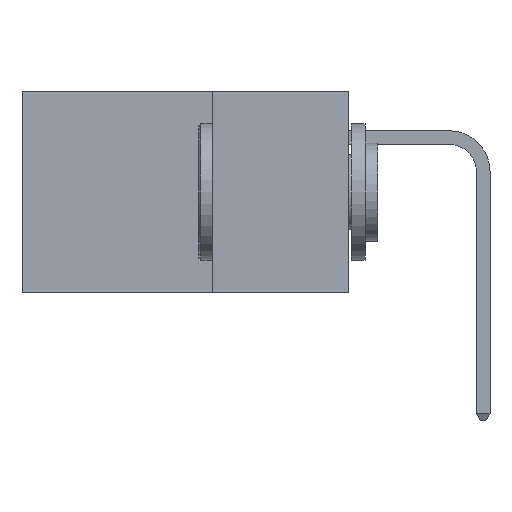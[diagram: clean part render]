
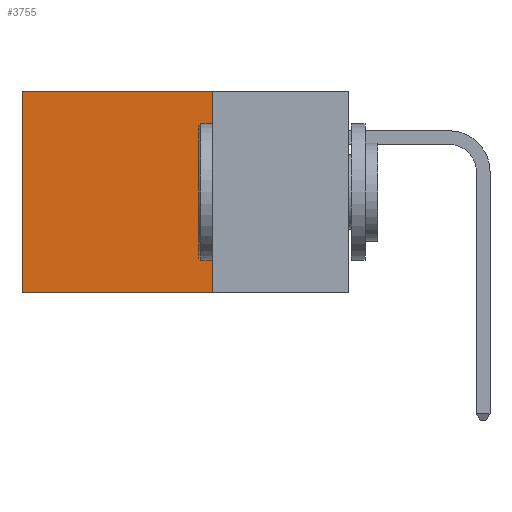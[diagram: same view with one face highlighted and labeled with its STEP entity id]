
A CAD part, left-side view. The second image highlights one B-rep face of the part: STEP entity #3755.
In plain terms, the highlighted planar face has unit normal (-1, 0, 0).
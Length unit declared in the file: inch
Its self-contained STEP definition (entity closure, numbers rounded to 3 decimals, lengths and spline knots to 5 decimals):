
#157 = VECTOR ( 'NONE', #552, 39.37008 ) ;
#552 = DIRECTION ( 'NONE',  ( 0., 0., -1. ) ) ;
#764 = LINE ( 'NONE', #7407, #3009 ) ;
#1059 = LINE ( 'NONE', #9791, #10030 ) ;
#1377 = VERTEX_POINT ( 'NONE', #9768 ) ;
#2729 = DIRECTION ( 'NONE',  ( 1., 0., 0. ) ) ;
#2749 = LINE ( 'NONE', #8305, #157 ) ;
#2848 = ORIENTED_EDGE ( 'NONE', *, *, #8945, .T. ) ;
#2862 = ORIENTED_EDGE ( 'NONE', *, *, #9578, .F. ) ;
#2917 = ORIENTED_EDGE ( 'NONE', *, *, #7736, .F. ) ;
#2971 = ORIENTED_EDGE ( 'NONE', *, *, #7416, .T. ) ;
#3009 = VECTOR ( 'NONE', #3635, 39.37008 ) ;
#3179 = VERTEX_POINT ( 'NONE', #8625 ) ;
#3292 = DIRECTION ( 'NONE',  ( 0., 0., -1. ) ) ;
#3604 = CARTESIAN_POINT ( 'NONE',  ( 0.2875, 0.25, 0. ) ) ;
#3635 = DIRECTION ( 'NONE',  ( 0., 0., -1. ) ) ;
#3755 = ADVANCED_FACE ( 'NONE', ( #9811 ), #4297, .F. ) ;
#4177 = VERTEX_POINT ( 'NONE', #10307 ) ;
#4297 = PLANE ( 'NONE',  #6810 ) ;
#4434 = VECTOR ( 'NONE', #9743, 39.37008 ) ;
#6696 = LINE ( 'NONE', #9763, #4434 ) ;
#6810 = AXIS2_PLACEMENT_3D ( 'NONE', #3604, #2729, #3292 ) ;
#7407 = CARTESIAN_POINT ( 'NONE',  ( 0.2875, 0.6, 0. ) ) ;
#7416 = EDGE_CURVE ( 'NONE', #9437, #3179, #6696, .T. ) ;
#7736 = EDGE_CURVE ( 'NONE', #9437, #4177, #2749, .T. ) ;
#8305 = CARTESIAN_POINT ( 'NONE',  ( 0.2875, 0.25, 0. ) ) ;
#8625 = CARTESIAN_POINT ( 'NONE',  ( 0.2875, 0.6, 0. ) ) ;
#8945 = EDGE_CURVE ( 'NONE', #3179, #1377, #764, .T. ) ;
#9092 = DIRECTION ( 'NONE',  ( 0., 1., 0. ) ) ;
#9230 = EDGE_LOOP ( 'NONE', ( #2848, #2862, #2917, #2971 ) ) ;
#9437 = VERTEX_POINT ( 'NONE', #10327 ) ;
#9578 = EDGE_CURVE ( 'NONE', #4177, #1377, #1059, .T. ) ;
#9743 = DIRECTION ( 'NONE',  ( 0., 1., 0. ) ) ;
#9763 = CARTESIAN_POINT ( 'NONE',  ( 0.2875, 0.25, 0. ) ) ;
#9768 = CARTESIAN_POINT ( 'NONE',  ( 0.2875, 0.6, -0.37 ) ) ;
#9791 = CARTESIAN_POINT ( 'NONE',  ( 0.2875, 0.25, -0.37 ) ) ;
#9811 = FACE_OUTER_BOUND ( 'NONE', #9230, .T. ) ;
#10030 = VECTOR ( 'NONE', #9092, 39.37008 ) ;
#10307 = CARTESIAN_POINT ( 'NONE',  ( 0.2875, 0.25, -0.37 ) ) ;
#10327 = CARTESIAN_POINT ( 'NONE',  ( 0.2875, 0.25, 0. ) ) ;
